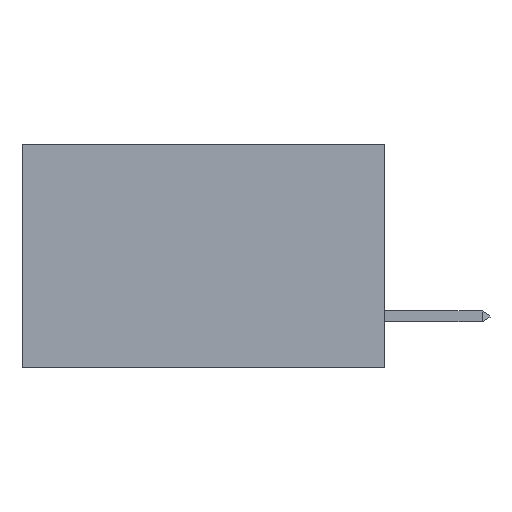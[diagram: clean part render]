
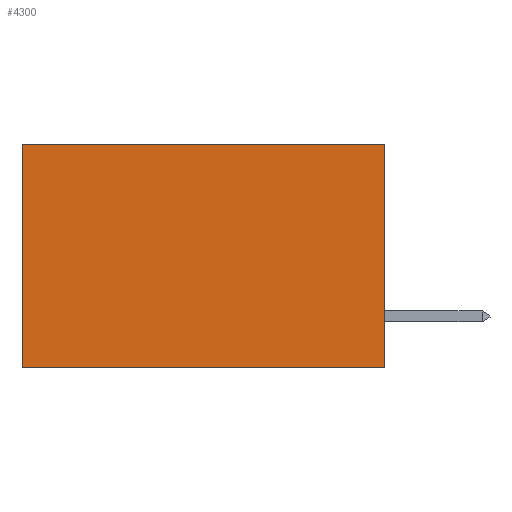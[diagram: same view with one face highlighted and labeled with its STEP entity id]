
A CAD part, left-side view. The second image highlights one B-rep face of the part: STEP entity #4300.
In plain terms, the highlighted planar face has unit normal (-1, 0, 0).
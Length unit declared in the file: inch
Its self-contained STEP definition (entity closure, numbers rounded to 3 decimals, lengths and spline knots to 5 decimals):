
#168 = VECTOR ( 'NONE', #7905, 39.37008 ) ;
#1663 = VECTOR ( 'NONE', #5066, 39.37008 ) ;
#1748 = EDGE_LOOP ( 'NONE', ( #11618, #6602, #5551, #6156 ) ) ;
#2455 = AXIS2_PLACEMENT_3D ( 'NONE', #9156, #9466, #8177 ) ;
#2693 = LINE ( 'NONE', #6996, #168 ) ;
#4062 = CARTESIAN_POINT ( 'NONE',  ( 0.2875, 0., 0. ) ) ;
#4300 = ADVANCED_FACE ( 'NONE', ( #10143 ), #10582, .F. ) ;
#4367 = VERTEX_POINT ( 'NONE', #9910 ) ;
#5005 = VERTEX_POINT ( 'NONE', #11114 ) ;
#5066 = DIRECTION ( 'NONE',  ( 0., 0., -1. ) ) ;
#5551 = ORIENTED_EDGE ( 'NONE', *, *, #11407, .F. ) ;
#5629 = CARTESIAN_POINT ( 'NONE',  ( 0.2875, 0.6, 0. ) ) ;
#6042 = VECTOR ( 'NONE', #10298, 39.37008 ) ;
#6156 = ORIENTED_EDGE ( 'NONE', *, *, #7637, .T. ) ;
#6602 = ORIENTED_EDGE ( 'NONE', *, *, #10107, .F. ) ;
#6680 = LINE ( 'NONE', #4062, #1663 ) ;
#6957 = CARTESIAN_POINT ( 'NONE',  ( 0.2875, 0.6, -0.37 ) ) ;
#6996 = CARTESIAN_POINT ( 'NONE',  ( 0.2875, 0., -0.37 ) ) ;
#7014 = VERTEX_POINT ( 'NONE', #6957 ) ;
#7637 = EDGE_CURVE ( 'NONE', #4367, #9268, #10352, .T. ) ;
#7753 = CARTESIAN_POINT ( 'NONE',  ( 0.2875, 0., 0. ) ) ;
#7905 = DIRECTION ( 'NONE',  ( 0., 1., 0. ) ) ;
#8177 = DIRECTION ( 'NONE',  ( 0., 0., -1. ) ) ;
#9156 = CARTESIAN_POINT ( 'NONE',  ( 0.2875, 0., 0. ) ) ;
#9268 = VERTEX_POINT ( 'NONE', #10539 ) ;
#9361 = VECTOR ( 'NONE', #10005, 39.37008 ) ;
#9466 = DIRECTION ( 'NONE',  ( 1., 0., 0. ) ) ;
#9621 = LINE ( 'NONE', #5629, #9361 ) ;
#9910 = CARTESIAN_POINT ( 'NONE',  ( 0.2875, 0., 0. ) ) ;
#10005 = DIRECTION ( 'NONE',  ( 0., 0., -1. ) ) ;
#10107 = EDGE_CURVE ( 'NONE', #5005, #7014, #2693, .T. ) ;
#10143 = FACE_OUTER_BOUND ( 'NONE', #1748, .T. ) ;
#10298 = DIRECTION ( 'NONE',  ( 0., 1., 0. ) ) ;
#10352 = LINE ( 'NONE', #7753, #6042 ) ;
#10539 = CARTESIAN_POINT ( 'NONE',  ( 0.2875, 0.6, 0. ) ) ;
#10582 = PLANE ( 'NONE',  #2455 ) ;
#11114 = CARTESIAN_POINT ( 'NONE',  ( 0.2875, 0., -0.37 ) ) ;
#11236 = EDGE_CURVE ( 'NONE', #9268, #7014, #9621, .T. ) ;
#11407 = EDGE_CURVE ( 'NONE', #4367, #5005, #6680, .T. ) ;
#11618 = ORIENTED_EDGE ( 'NONE', *, *, #11236, .T. ) ;
